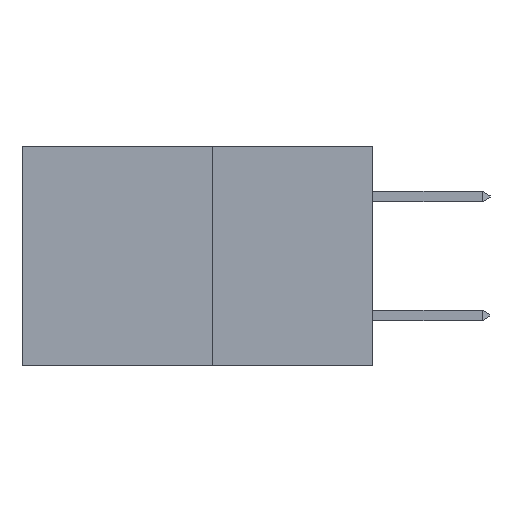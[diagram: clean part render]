
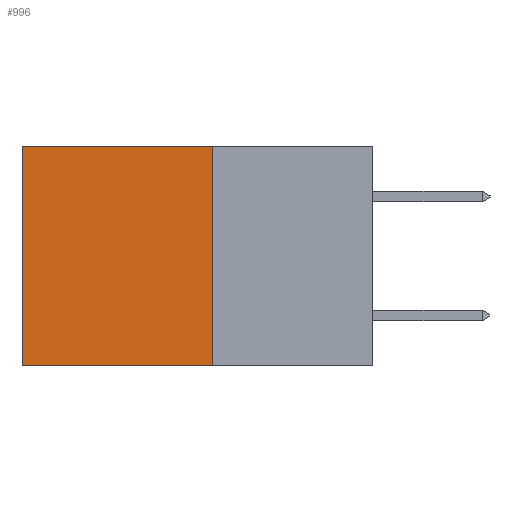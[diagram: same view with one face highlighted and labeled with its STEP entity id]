
A CAD part, left-side view. The second image highlights one B-rep face of the part: STEP entity #996.
In plain terms, the highlighted planar face has unit normal (-1, 0, 0).
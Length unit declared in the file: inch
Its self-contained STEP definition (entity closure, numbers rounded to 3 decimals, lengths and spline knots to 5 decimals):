
#268 = VERTEX_POINT ( 'NONE', #1606 ) ;
#285 = CARTESIAN_POINT ( 'NONE',  ( 0.277, 0.27, -0.37 ) ) ;
#430 = LINE ( 'NONE', #10366, #7125 ) ;
#600 = PLANE ( 'NONE',  #7846 ) ;
#996 = ADVANCED_FACE ( 'NONE', ( #3904 ), #600, .F. ) ;
#1204 = VECTOR ( 'NONE', #1568, 39.37008 ) ;
#1247 = VECTOR ( 'NONE', #9760, 39.37008 ) ;
#1568 = DIRECTION ( 'NONE',  ( 0., 0., -1. ) ) ;
#1606 = CARTESIAN_POINT ( 'NONE',  ( 0.277, 0.59, 0. ) ) ;
#1872 = LINE ( 'NONE', #7563, #10849 ) ;
#2341 = EDGE_CURVE ( 'NONE', #3296, #2699, #10477, .T. ) ;
#2699 = VERTEX_POINT ( 'NONE', #7398 ) ;
#3296 = VERTEX_POINT ( 'NONE', #285 ) ;
#3733 = DIRECTION ( 'NONE',  ( 0., 0., -1. ) ) ;
#3904 = FACE_OUTER_BOUND ( 'NONE', #4368, .T. ) ;
#4259 = EDGE_CURVE ( 'NONE', #6500, #3296, #8162, .T. ) ;
#4368 = EDGE_LOOP ( 'NONE', ( #6659, #9124, #5869, #10073 ) ) ;
#5869 = ORIENTED_EDGE ( 'NONE', *, *, #4259, .F. ) ;
#5896 = CARTESIAN_POINT ( 'NONE',  ( 0.277, 0.27, -0.37 ) ) ;
#5935 = CARTESIAN_POINT ( 'NONE',  ( 0.277, 0.27, -0.37 ) ) ;
#6500 = VERTEX_POINT ( 'NONE', #6761 ) ;
#6659 = ORIENTED_EDGE ( 'NONE', *, *, #10823, .T. ) ;
#6761 = CARTESIAN_POINT ( 'NONE',  ( 0.277, 0.27, 0. ) ) ;
#7125 = VECTOR ( 'NONE', #10000, 39.37008 ) ;
#7278 = EDGE_CURVE ( 'NONE', #6500, #268, #430, .T. ) ;
#7398 = CARTESIAN_POINT ( 'NONE',  ( 0.277, 0.59, -0.37 ) ) ;
#7563 = CARTESIAN_POINT ( 'NONE',  ( 0.277, 0.59, -0.37 ) ) ;
#7846 = AXIS2_PLACEMENT_3D ( 'NONE', #5896, #10300, #3733 ) ;
#8162 = LINE ( 'NONE', #5935, #1204 ) ;
#9124 = ORIENTED_EDGE ( 'NONE', *, *, #2341, .F. ) ;
#9760 = DIRECTION ( 'NONE',  ( 0., 1., 0. ) ) ;
#9999 = CARTESIAN_POINT ( 'NONE',  ( 0.277, 0.27, -0.37 ) ) ;
#10000 = DIRECTION ( 'NONE',  ( 0., 1., 0. ) ) ;
#10073 = ORIENTED_EDGE ( 'NONE', *, *, #7278, .T. ) ;
#10193 = DIRECTION ( 'NONE',  ( 0., 0., -1. ) ) ;
#10300 = DIRECTION ( 'NONE',  ( 1., 0., 0. ) ) ;
#10366 = CARTESIAN_POINT ( 'NONE',  ( 0.277, 0.27, 0. ) ) ;
#10477 = LINE ( 'NONE', #9999, #1247 ) ;
#10823 = EDGE_CURVE ( 'NONE', #268, #2699, #1872, .T. ) ;
#10849 = VECTOR ( 'NONE', #10193, 39.37008 ) ;
